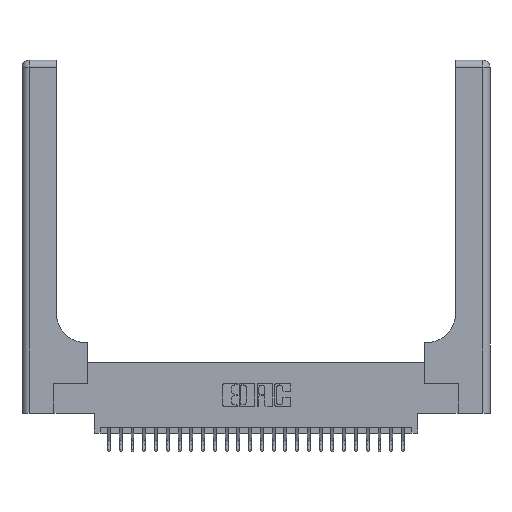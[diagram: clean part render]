
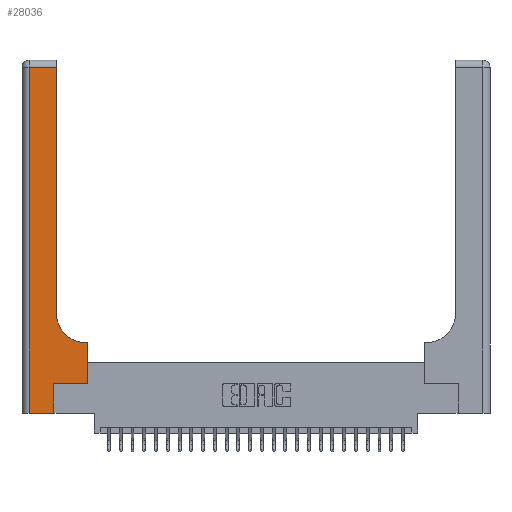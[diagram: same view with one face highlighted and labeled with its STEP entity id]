
A CAD part, top view. The second image highlights one B-rep face of the part: STEP entity #28036.
In plain terms, the highlighted planar face has unit normal (0, 0, 1).
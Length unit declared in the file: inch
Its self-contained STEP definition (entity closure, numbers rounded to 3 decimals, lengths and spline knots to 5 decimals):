
#38 = LINE ( 'NONE', #1049, #20437 ) ;
#168 = CIRCLE ( 'NONE', #15594, 0.25 ) ;
#305 = CARTESIAN_POINT ( 'NONE',  ( 0.269, 0.25, 0.37 ) ) ;
#527 = CARTESIAN_POINT ( 'NONE',  ( 0.5585, 0.6, 0.37 ) ) ;
#914 = LINE ( 'NONE', #3185, #25035 ) ;
#1049 = CARTESIAN_POINT ( 'NONE',  ( 0.06, 3., 0.37 ) ) ;
#1642 = LINE ( 'NONE', #3017, #16266 ) ;
#1851 = DIRECTION ( 'NONE',  ( 0., 0., -1. ) ) ;
#2032 = LINE ( 'NONE', #19958, #23818 ) ;
#2663 = VERTEX_POINT ( 'NONE', #21769 ) ;
#2718 = EDGE_CURVE ( 'NONE', #17100, #13274, #9475, .T. ) ;
#2759 = EDGE_CURVE ( 'NONE', #24948, #4974, #17344, .T. ) ;
#3017 = CARTESIAN_POINT ( 'NONE',  ( 0.269, 0., 0.37 ) ) ;
#3185 = CARTESIAN_POINT ( 'NONE',  ( 0., 0., 0.37 ) ) ;
#3435 = EDGE_CURVE ( 'NONE', #18709, #17100, #1642, .T. ) ;
#3825 = PLANE ( 'NONE',  #22208 ) ;
#3960 = VERTEX_POINT ( 'NONE', #8022 ) ;
#4435 = CARTESIAN_POINT ( 'NONE',  ( 0.2915, 0.6, 0.37 ) ) ;
#4523 = ORIENTED_EDGE ( 'NONE', *, *, #27013, .T. ) ;
#4897 = FACE_OUTER_BOUND ( 'NONE', #7343, .T. ) ;
#4974 = VERTEX_POINT ( 'NONE', #9090 ) ;
#5361 = DIRECTION ( 'NONE',  ( 0., 1., 0. ) ) ;
#5916 = EDGE_CURVE ( 'NONE', #8287, #3960, #25192, .T. ) ;
#6091 = EDGE_CURVE ( 'NONE', #3960, #2663, #38, .T. ) ;
#6128 = VECTOR ( 'NONE', #19764, 39.37008 ) ;
#6171 = ORIENTED_EDGE ( 'NONE', *, *, #5916, .T. ) ;
#6648 = VECTOR ( 'NONE', #9780, 39.37008 ) ;
#7343 = EDGE_LOOP ( 'NONE', ( #7930, #6171, #18250, #17730, #25026, #16983, #24247, #16119, #4523 ) ) ;
#7788 = DIRECTION ( 'NONE',  ( 0., -1., 0. ) ) ;
#7930 = ORIENTED_EDGE ( 'NONE', *, *, #21743, .T. ) ;
#8022 = CARTESIAN_POINT ( 'NONE',  ( 0.06, 2.94, 0.37 ) ) ;
#8287 = VERTEX_POINT ( 'NONE', #23127 ) ;
#8658 = DIRECTION ( 'NONE',  ( 1., 0., 0. ) ) ;
#8748 = CARTESIAN_POINT ( 'NONE',  ( 0.5415, 0.85, 0.37 ) ) ;
#9090 = CARTESIAN_POINT ( 'NONE',  ( 0.5415, 0.6, 0.37 ) ) ;
#9475 = LINE ( 'NONE', #305, #14959 ) ;
#9542 = EDGE_CURVE ( 'NONE', #2663, #18709, #914, .T. ) ;
#9657 = CARTESIAN_POINT ( 'NONE',  ( 0.269, 0.25, 0.37 ) ) ;
#9780 = DIRECTION ( 'NONE',  ( 0., 1., 0. ) ) ;
#10151 = VECTOR ( 'NONE', #21878, 39.37008 ) ;
#13274 = VERTEX_POINT ( 'NONE', #21168 ) ;
#13935 = DIRECTION ( 'NONE',  ( 0., 1., 0. ) ) ;
#14504 = LINE ( 'NONE', #20542, #6648 ) ;
#14946 = EDGE_CURVE ( 'NONE', #13274, #24948, #2032, .T. ) ;
#14959 = VECTOR ( 'NONE', #17318, 39.37008 ) ;
#15587 = CARTESIAN_POINT ( 'NONE',  ( 0.2915, 0.85, 0.37 ) ) ;
#15594 = AXIS2_PLACEMENT_3D ( 'NONE', #8748, #17515, #8658 ) ;
#16119 = ORIENTED_EDGE ( 'NONE', *, *, #2759, .T. ) ;
#16266 = VECTOR ( 'NONE', #13935, 39.37008 ) ;
#16983 = ORIENTED_EDGE ( 'NONE', *, *, #2718, .T. ) ;
#17100 = VERTEX_POINT ( 'NONE', #9657 ) ;
#17318 = DIRECTION ( 'NONE',  ( 1., 0., 0. ) ) ;
#17344 = LINE ( 'NONE', #4435, #10151 ) ;
#17515 = DIRECTION ( 'NONE',  ( 0., 0., -1. ) ) ;
#17730 = ORIENTED_EDGE ( 'NONE', *, *, #9542, .T. ) ;
#18250 = ORIENTED_EDGE ( 'NONE', *, *, #6091, .T. ) ;
#18709 = VERTEX_POINT ( 'NONE', #26878 ) ;
#19764 = DIRECTION ( 'NONE',  ( -1., 0., 0. ) ) ;
#19958 = CARTESIAN_POINT ( 'NONE',  ( 0.5585, 0.25, 0.37 ) ) ;
#20437 = VECTOR ( 'NONE', #7788, 39.37008 ) ;
#20542 = CARTESIAN_POINT ( 'NONE',  ( 0.2915, 3., 0.37 ) ) ;
#21168 = CARTESIAN_POINT ( 'NONE',  ( 0.5585, 0.25, 0.37 ) ) ;
#21743 = EDGE_CURVE ( 'NONE', #25664, #8287, #14504, .T. ) ;
#21769 = CARTESIAN_POINT ( 'NONE',  ( 0.06, 0., 0.37 ) ) ;
#21878 = DIRECTION ( 'NONE',  ( -1., 0., 0. ) ) ;
#22208 = AXIS2_PLACEMENT_3D ( 'NONE', #23457, #1851, #25406 ) ;
#22830 = DIRECTION ( 'NONE',  ( 1., 0., 0. ) ) ;
#23127 = CARTESIAN_POINT ( 'NONE',  ( 0.2915, 2.94, 0.37 ) ) ;
#23457 = CARTESIAN_POINT ( 'NONE',  ( 0., 3., 0.37 ) ) ;
#23764 = CARTESIAN_POINT ( 'NONE',  ( 0., 2.94, 0.37 ) ) ;
#23818 = VECTOR ( 'NONE', #5361, 39.37008 ) ;
#24247 = ORIENTED_EDGE ( 'NONE', *, *, #14946, .T. ) ;
#24948 = VERTEX_POINT ( 'NONE', #527 ) ;
#25026 = ORIENTED_EDGE ( 'NONE', *, *, #3435, .T. ) ;
#25035 = VECTOR ( 'NONE', #22830, 39.37008 ) ;
#25192 = LINE ( 'NONE', #23764, #6128 ) ;
#25406 = DIRECTION ( 'NONE',  ( -1., 0., 0. ) ) ;
#25664 = VERTEX_POINT ( 'NONE', #15587 ) ;
#26878 = CARTESIAN_POINT ( 'NONE',  ( 0.269, 0., 0.37 ) ) ;
#27013 = EDGE_CURVE ( 'NONE', #4974, #25664, #168, .T. ) ;
#28036 = ADVANCED_FACE ( 'NONE', ( #4897 ), #3825, .F. ) ;
